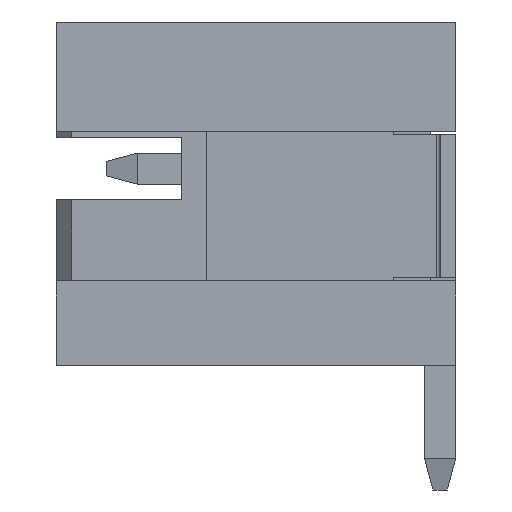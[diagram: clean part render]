
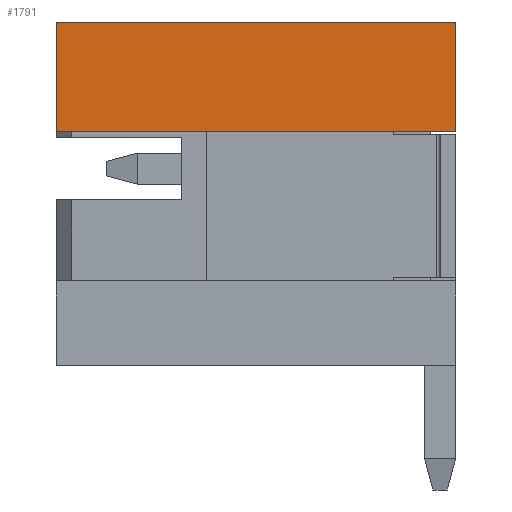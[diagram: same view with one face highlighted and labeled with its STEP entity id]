
A CAD part, left-side view. The second image highlights one B-rep face of the part: STEP entity #1791.
In plain terms, the highlighted planar face has unit normal (-1, 0, 0).
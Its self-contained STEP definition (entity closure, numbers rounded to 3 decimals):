
#247 = LINE ( 'NONE', #1721, #1266 ) ;
#389 = CARTESIAN_POINT ( 'NONE',  ( -3., 0., 0.6 ) ) ;
#546 = VERTEX_POINT ( 'NONE', #6717 ) ;
#655 = ORIENTED_EDGE ( 'NONE', *, *, #6665, .F. ) ;
#938 = CARTESIAN_POINT ( 'NONE',  ( -3., 0., 0. ) ) ;
#1004 = DIRECTION ( 'NONE',  ( 0., 1., 0. ) ) ;
#1266 = VECTOR ( 'NONE', #3970, 1000. ) ;
#1280 = EDGE_CURVE ( 'NONE', #1861, #4557, #247, .T. ) ;
#1711 = FACE_OUTER_BOUND ( 'NONE', #1889, .T. ) ;
#1721 = CARTESIAN_POINT ( 'NONE',  ( -3., 0., 2.35 ) ) ;
#1791 = ADVANCED_FACE ( 'NONE', ( #1711 ), #5563, .F. ) ;
#1861 = VERTEX_POINT ( 'NONE', #5640 ) ;
#1889 = EDGE_LOOP ( 'NONE', ( #655, #4888, #7352, #5168 ) ) ;
#1917 = VECTOR ( 'NONE', #1004, 1000. ) ;
#1994 = CARTESIAN_POINT ( 'NONE',  ( -3., 6.4, 2.35 ) ) ;
#3040 = EDGE_CURVE ( 'NONE', #7432, #1861, #5979, .T. ) ;
#3363 = AXIS2_PLACEMENT_3D ( 'NONE', #938, #6161, #7318 ) ;
#3970 = DIRECTION ( 'NONE',  ( 0., 0., -1. ) ) ;
#4019 = CARTESIAN_POINT ( 'NONE',  ( -3., 6.4, 2.35 ) ) ;
#4054 = CARTESIAN_POINT ( 'NONE',  ( -3., 6.4, 2.35 ) ) ;
#4274 = LINE ( 'NONE', #4019, #7266 ) ;
#4309 = CARTESIAN_POINT ( 'NONE',  ( -3., 0., 0.6 ) ) ;
#4557 = VERTEX_POINT ( 'NONE', #4309 ) ;
#4888 = ORIENTED_EDGE ( 'NONE', *, *, #5313, .F. ) ;
#5168 = ORIENTED_EDGE ( 'NONE', *, *, #3040, .F. ) ;
#5313 = EDGE_CURVE ( 'NONE', #4557, #546, #6902, .T. ) ;
#5563 = PLANE ( 'NONE',  #3363 ) ;
#5640 = CARTESIAN_POINT ( 'NONE',  ( -3., 0., 2.35 ) ) ;
#5774 = DIRECTION ( 'NONE',  ( 0., 0., 1. ) ) ;
#5979 = LINE ( 'NONE', #1994, #6541 ) ;
#6161 = DIRECTION ( 'NONE',  ( 1., 0., 0. ) ) ;
#6541 = VECTOR ( 'NONE', #7301, 1000. ) ;
#6665 = EDGE_CURVE ( 'NONE', #546, #7432, #4274, .T. ) ;
#6717 = CARTESIAN_POINT ( 'NONE',  ( -3., 6.4, 0.6 ) ) ;
#6902 = LINE ( 'NONE', #389, #1917 ) ;
#7266 = VECTOR ( 'NONE', #5774, 1000. ) ;
#7301 = DIRECTION ( 'NONE',  ( 0., -1., 0. ) ) ;
#7318 = DIRECTION ( 'NONE',  ( 0., 0., -1. ) ) ;
#7352 = ORIENTED_EDGE ( 'NONE', *, *, #1280, .F. ) ;
#7432 = VERTEX_POINT ( 'NONE', #4054 ) ;
